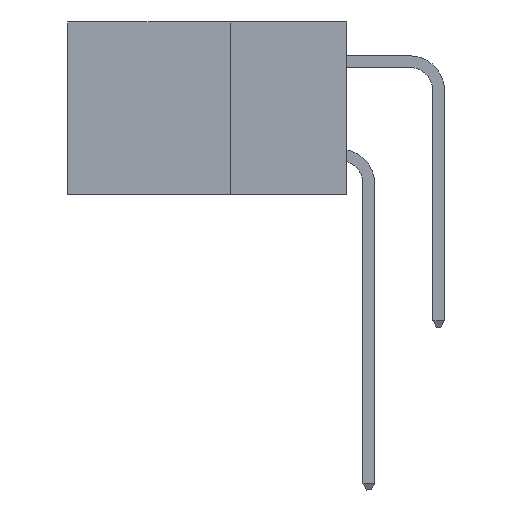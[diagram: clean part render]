
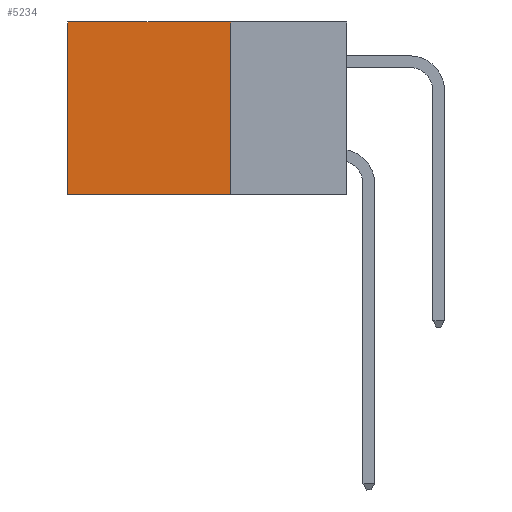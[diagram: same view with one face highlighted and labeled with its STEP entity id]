
A CAD part, left-side view. The second image highlights one B-rep face of the part: STEP entity #5234.
In plain terms, the highlighted planar face has unit normal (-1, 0, 0).
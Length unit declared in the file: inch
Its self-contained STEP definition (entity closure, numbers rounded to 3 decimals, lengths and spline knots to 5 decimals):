
#851 = VECTOR ( 'NONE', #18423, 39.37008 ) ;
#900 = LINE ( 'NONE', #12327, #18236 ) ;
#1436 = CARTESIAN_POINT ( 'NONE',  ( 0.2875, 0.25, 0. ) ) ;
#1501 = CARTESIAN_POINT ( 'NONE',  ( 0.2875, 0.25, 0. ) ) ;
#1529 = FACE_OUTER_BOUND ( 'NONE', #21249, .T. ) ;
#1831 = EDGE_CURVE ( 'NONE', #19483, #17895, #16757, .T. ) ;
#2932 = ORIENTED_EDGE ( 'NONE', *, *, #6908, .T. ) ;
#3190 = DIRECTION ( 'NONE',  ( 1., 0., 0. ) ) ;
#5234 = ADVANCED_FACE ( 'NONE', ( #1529 ), #21413, .F. ) ;
#5297 = CARTESIAN_POINT ( 'NONE',  ( 0.2875, 0.6, -0.37 ) ) ;
#5802 = CARTESIAN_POINT ( 'NONE',  ( 0.2875, 0.6, 0. ) ) ;
#5937 = DIRECTION ( 'NONE',  ( 0., 0., -1. ) ) ;
#6908 = EDGE_CURVE ( 'NONE', #7272, #19483, #900, .T. ) ;
#6995 = DIRECTION ( 'NONE',  ( 0., 0., -1. ) ) ;
#7272 = VERTEX_POINT ( 'NONE', #1501 ) ;
#7705 = LINE ( 'NONE', #10400, #20383 ) ;
#8261 = VERTEX_POINT ( 'NONE', #8667 ) ;
#8667 = CARTESIAN_POINT ( 'NONE',  ( 0.2875, 0.25, -0.37 ) ) ;
#8726 = AXIS2_PLACEMENT_3D ( 'NONE', #1436, #3190, #14886 ) ;
#9066 = DIRECTION ( 'NONE',  ( 0., 1., 0. ) ) ;
#9281 = ORIENTED_EDGE ( 'NONE', *, *, #17921, .F. ) ;
#10400 = CARTESIAN_POINT ( 'NONE',  ( 0.2875, 0.25, 0. ) ) ;
#10442 = LINE ( 'NONE', #11719, #851 ) ;
#11285 = ORIENTED_EDGE ( 'NONE', *, *, #1831, .T. ) ;
#11719 = CARTESIAN_POINT ( 'NONE',  ( 0.2875, 0.25, -0.37 ) ) ;
#12327 = CARTESIAN_POINT ( 'NONE',  ( 0.2875, 0.25, 0. ) ) ;
#12357 = VECTOR ( 'NONE', #5937, 39.37008 ) ;
#14295 = EDGE_CURVE ( 'NONE', #8261, #17895, #10442, .T. ) ;
#14886 = DIRECTION ( 'NONE',  ( 0., 0., -1. ) ) ;
#16223 = ORIENTED_EDGE ( 'NONE', *, *, #14295, .F. ) ;
#16757 = LINE ( 'NONE', #5802, #12357 ) ;
#17895 = VERTEX_POINT ( 'NONE', #5297 ) ;
#17921 = EDGE_CURVE ( 'NONE', #7272, #8261, #7705, .T. ) ;
#18236 = VECTOR ( 'NONE', #9066, 39.37008 ) ;
#18423 = DIRECTION ( 'NONE',  ( 0., 1., 0. ) ) ;
#19483 = VERTEX_POINT ( 'NONE', #21334 ) ;
#20383 = VECTOR ( 'NONE', #6995, 39.37008 ) ;
#21249 = EDGE_LOOP ( 'NONE', ( #11285, #16223, #9281, #2932 ) ) ;
#21334 = CARTESIAN_POINT ( 'NONE',  ( 0.2875, 0.6, 0. ) ) ;
#21413 = PLANE ( 'NONE',  #8726 ) ;
